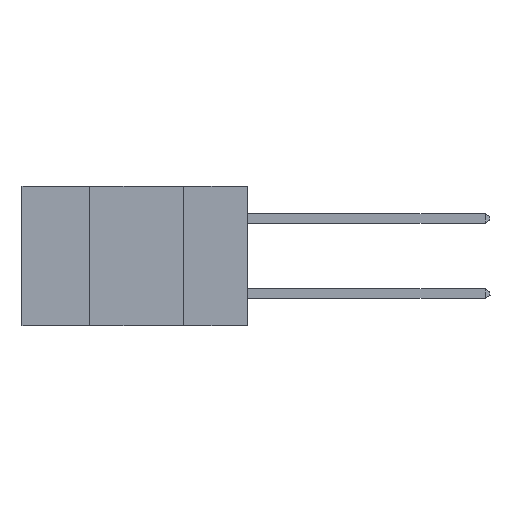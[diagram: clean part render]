
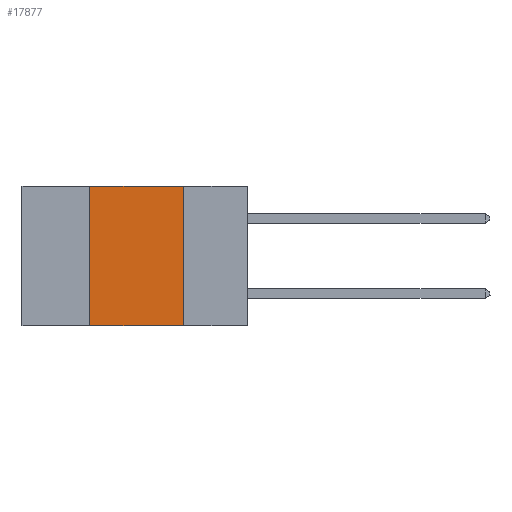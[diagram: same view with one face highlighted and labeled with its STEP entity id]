
A CAD part, left-side view. The second image highlights one B-rep face of the part: STEP entity #17877.
In plain terms, the highlighted planar face has unit normal (-1, 0, 0).
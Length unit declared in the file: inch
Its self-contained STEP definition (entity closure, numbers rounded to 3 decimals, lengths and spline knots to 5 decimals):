
#490 = DIRECTION ( 'NONE',  ( 0., -1., 0. ) ) ;
#1459 = CARTESIAN_POINT ( 'NONE',  ( 0., 0.42, -0.37 ) ) ;
#1498 = EDGE_CURVE ( 'NONE', #19586, #8866, #20550, .T. ) ;
#1549 = CARTESIAN_POINT ( 'NONE',  ( 0., 0.17, 0. ) ) ;
#2419 = PLANE ( 'NONE',  #16148 ) ;
#2669 = EDGE_CURVE ( 'NONE', #21004, #6071, #13933, .T. ) ;
#4022 = LINE ( 'NONE', #25495, #15750 ) ;
#4281 = CARTESIAN_POINT ( 'NONE',  ( 0., 0.17, 0. ) ) ;
#5637 = VECTOR ( 'NONE', #17637, 39.37008 ) ;
#6071 = VERTEX_POINT ( 'NONE', #15718 ) ;
#8235 = CARTESIAN_POINT ( 'NONE',  ( 0., 0.6, -0.37 ) ) ;
#8466 = LINE ( 'NONE', #8235, #18694 ) ;
#8638 = DIRECTION ( 'NONE',  ( 0., 0., -1. ) ) ;
#8866 = VERTEX_POINT ( 'NONE', #14900 ) ;
#10214 = ORIENTED_EDGE ( 'NONE', *, *, #13910, .T. ) ;
#12174 = EDGE_LOOP ( 'NONE', ( #17167, #21258, #24231, #10214 ) ) ;
#12421 = DIRECTION ( 'NONE',  ( 1., 0., 0. ) ) ;
#13910 = EDGE_CURVE ( 'NONE', #21004, #8866, #8466, .T. ) ;
#13933 = LINE ( 'NONE', #21979, #23542 ) ;
#14493 = CARTESIAN_POINT ( 'NONE',  ( 0., 0.6, 0. ) ) ;
#14900 = CARTESIAN_POINT ( 'NONE',  ( 0., 0.17, -0.37 ) ) ;
#15417 = DIRECTION ( 'NONE',  ( 0., -1., 0. ) ) ;
#15718 = CARTESIAN_POINT ( 'NONE',  ( 0., 0.42, 0. ) ) ;
#15750 = VECTOR ( 'NONE', #15417, 39.37008 ) ;
#16095 = DIRECTION ( 'NONE',  ( 0., 0., 1. ) ) ;
#16148 = AXIS2_PLACEMENT_3D ( 'NONE', #14493, #12421, #8638 ) ;
#17014 = FACE_OUTER_BOUND ( 'NONE', #12174, .T. ) ;
#17167 = ORIENTED_EDGE ( 'NONE', *, *, #1498, .F. ) ;
#17637 = DIRECTION ( 'NONE',  ( 0., 0., -1. ) ) ;
#17877 = ADVANCED_FACE ( 'NONE', ( #17014 ), #2419, .F. ) ;
#18694 = VECTOR ( 'NONE', #490, 39.37008 ) ;
#19586 = VERTEX_POINT ( 'NONE', #4281 ) ;
#20550 = LINE ( 'NONE', #1549, #5637 ) ;
#21004 = VERTEX_POINT ( 'NONE', #1459 ) ;
#21258 = ORIENTED_EDGE ( 'NONE', *, *, #23216, .F. ) ;
#21979 = CARTESIAN_POINT ( 'NONE',  ( 0., 0.42, 0. ) ) ;
#23216 = EDGE_CURVE ( 'NONE', #6071, #19586, #4022, .T. ) ;
#23542 = VECTOR ( 'NONE', #16095, 39.37008 ) ;
#24231 = ORIENTED_EDGE ( 'NONE', *, *, #2669, .F. ) ;
#25495 = CARTESIAN_POINT ( 'NONE',  ( 0., 0.6, 0. ) ) ;
